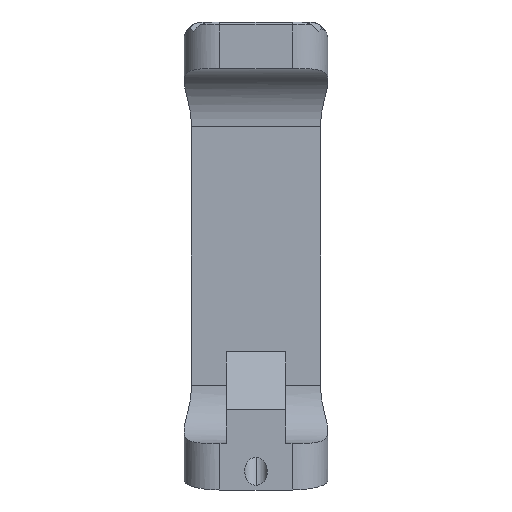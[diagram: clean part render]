
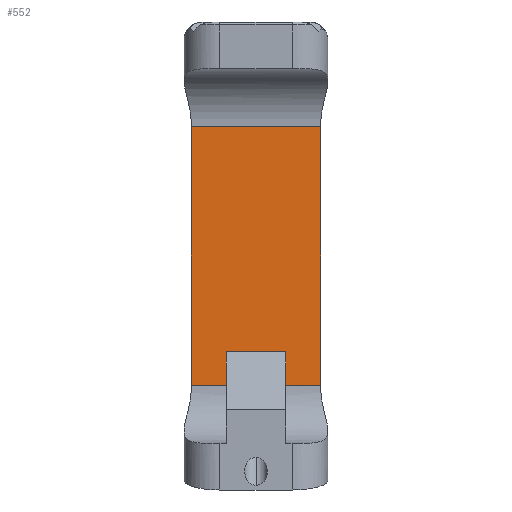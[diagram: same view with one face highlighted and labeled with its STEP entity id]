
A CAD part, left-side view. The second image highlights one B-rep face of the part: STEP entity #552.
In plain terms, the highlighted planar face has unit normal (-1, 0, 0).
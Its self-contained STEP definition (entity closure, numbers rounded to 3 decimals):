
#144 = CARTESIAN_POINT ( 'NONE',  ( 0.083, 4.299, 8.598 ) ) ;
#149 = DIRECTION ( 'NONE',  ( 0., -1., 0. ) ) ;
#175 = CARTESIAN_POINT ( 'NONE',  ( 0.083, 1.968, -8.598 ) ) ;
#198 = CARTESIAN_POINT ( 'NONE',  ( 0.083, -4.299, 4.299 ) ) ;
#211 = EDGE_CURVE ( 'NONE', #2438, #1400, #2685, .T. ) ;
#233 = DIRECTION ( 'NONE',  ( 1., 0., 0. ) ) ;
#234 = AXIS2_PLACEMENT_3D ( 'NONE', #1696, #233, #1936 ) ;
#269 = VERTEX_POINT ( 'NONE', #2342 ) ;
#280 = DIRECTION ( 'NONE',  ( 0., 1., 0. ) ) ;
#281 = EDGE_CURVE ( 'NONE', #300, #2438, #3070, .T. ) ;
#300 = VERTEX_POINT ( 'NONE', #2918 ) ;
#307 = FACE_OUTER_BOUND ( 'NONE', #1974, .T. ) ;
#377 = EDGE_CURVE ( 'NONE', #650, #269, #2855, .T. ) ;
#386 = VECTOR ( 'NONE', #2605, 1000. ) ;
#492 = DIRECTION ( 'NONE',  ( 0., -1., 0. ) ) ;
#508 = EDGE_CURVE ( 'NONE', #2141, #269, #2316, .T. ) ;
#552 = ADVANCED_FACE ( 'NONE', ( #307 ), #1448, .F. ) ;
#645 = LINE ( 'NONE', #2724, #3073 ) ;
#650 = VERTEX_POINT ( 'NONE', #1493 ) ;
#651 = EDGE_CURVE ( 'NONE', #2141, #1443, #2102, .T. ) ;
#977 = VECTOR ( 'NONE', #492, 1000. ) ;
#1009 = ORIENTED_EDGE ( 'NONE', *, *, #211, .T. ) ;
#1082 = LINE ( 'NONE', #2785, #2286 ) ;
#1098 = CARTESIAN_POINT ( 'NONE',  ( 0.083, 1.968, -6.369 ) ) ;
#1105 = ORIENTED_EDGE ( 'NONE', *, *, #2974, .T. ) ;
#1309 = VECTOR ( 'NONE', #280, 1000. ) ;
#1400 = VERTEX_POINT ( 'NONE', #1098 ) ;
#1443 = VERTEX_POINT ( 'NONE', #144 ) ;
#1448 = PLANE ( 'NONE',  #234 ) ;
#1457 = EDGE_CURVE ( 'NONE', #300, #1443, #1082, .T. ) ;
#1493 = CARTESIAN_POINT ( 'NONE',  ( 0.083, -1.968, -8.598 ) ) ;
#1557 = DIRECTION ( 'NONE',  ( 0., 0., -1. ) ) ;
#1696 = CARTESIAN_POINT ( 'NONE',  ( 0.083, 0., 8.598 ) ) ;
#1736 = CARTESIAN_POINT ( 'NONE',  ( 0.083, 0., 8.598 ) ) ;
#1799 = LINE ( 'NONE', #2183, #977 ) ;
#1804 = CARTESIAN_POINT ( 'NONE',  ( 0.083, -1.968, -6.369 ) ) ;
#1936 = DIRECTION ( 'NONE',  ( 0., 0., -1. ) ) ;
#1974 = EDGE_LOOP ( 'NONE', ( #1009, #1105, #2224, #2963, #2807, #2982, #2241, #2230 ) ) ;
#2000 = VECTOR ( 'NONE', #3000, 1000. ) ;
#2019 = CARTESIAN_POINT ( 'NONE',  ( 0.083, 1.968, -0.452 ) ) ;
#2082 = CARTESIAN_POINT ( 'NONE',  ( 0.083, 0., -8.598 ) ) ;
#2097 = DIRECTION ( 'NONE',  ( 0., -1., 0. ) ) ;
#2102 = LINE ( 'NONE', #1736, #1309 ) ;
#2141 = VERTEX_POINT ( 'NONE', #2463 ) ;
#2183 = CARTESIAN_POINT ( 'NONE',  ( 0.083, 0., -6.369 ) ) ;
#2224 = ORIENTED_EDGE ( 'NONE', *, *, #2826, .T. ) ;
#2230 = ORIENTED_EDGE ( 'NONE', *, *, #281, .T. ) ;
#2241 = ORIENTED_EDGE ( 'NONE', *, *, #1457, .F. ) ;
#2264 = VECTOR ( 'NONE', #149, 1000. ) ;
#2286 = VECTOR ( 'NONE', #3004, 1000. ) ;
#2316 = LINE ( 'NONE', #198, #386 ) ;
#2342 = CARTESIAN_POINT ( 'NONE',  ( 0.083, -4.299, -8.598 ) ) ;
#2438 = VERTEX_POINT ( 'NONE', #175 ) ;
#2463 = CARTESIAN_POINT ( 'NONE',  ( 0.083, -4.299, 8.598 ) ) ;
#2474 = VECTOR ( 'NONE', #2097, 1000. ) ;
#2546 = CARTESIAN_POINT ( 'NONE',  ( 0.083, 0., -8.598 ) ) ;
#2605 = DIRECTION ( 'NONE',  ( 0., 0., -1. ) ) ;
#2685 = LINE ( 'NONE', #2019, #2000 ) ;
#2724 = CARTESIAN_POINT ( 'NONE',  ( 0.083, -1.968, -0.452 ) ) ;
#2771 = VERTEX_POINT ( 'NONE', #1804 ) ;
#2785 = CARTESIAN_POINT ( 'NONE',  ( 0.083, 4.299, 4.299 ) ) ;
#2807 = ORIENTED_EDGE ( 'NONE', *, *, #508, .F. ) ;
#2826 = EDGE_CURVE ( 'NONE', #2771, #650, #645, .T. ) ;
#2855 = LINE ( 'NONE', #2082, #2264 ) ;
#2918 = CARTESIAN_POINT ( 'NONE',  ( 0.083, 4.299, -8.598 ) ) ;
#2963 = ORIENTED_EDGE ( 'NONE', *, *, #377, .T. ) ;
#2974 = EDGE_CURVE ( 'NONE', #1400, #2771, #1799, .T. ) ;
#2982 = ORIENTED_EDGE ( 'NONE', *, *, #651, .T. ) ;
#3000 = DIRECTION ( 'NONE',  ( 0., 0., 1. ) ) ;
#3004 = DIRECTION ( 'NONE',  ( 0., 0., 1. ) ) ;
#3070 = LINE ( 'NONE', #2546, #2474 ) ;
#3073 = VECTOR ( 'NONE', #1557, 1000. ) ;
